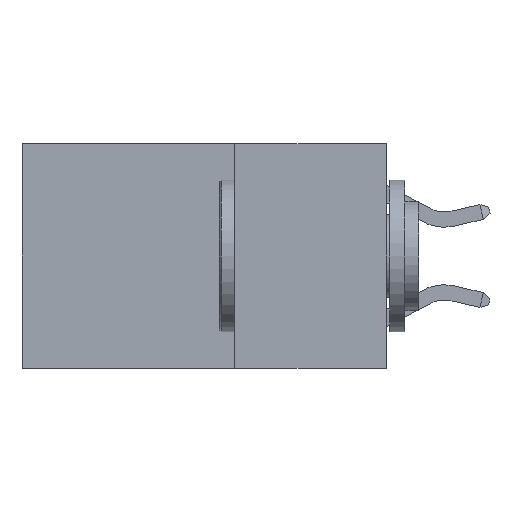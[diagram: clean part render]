
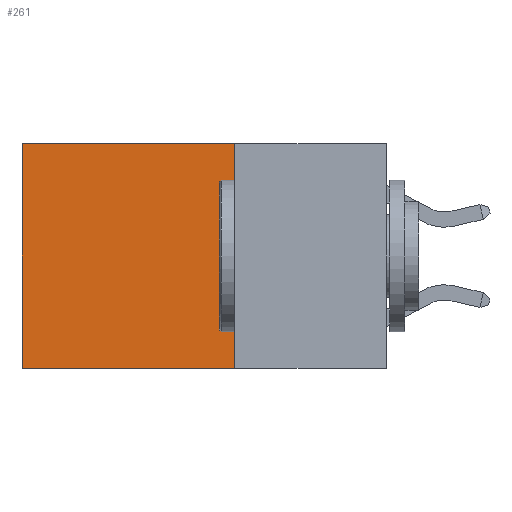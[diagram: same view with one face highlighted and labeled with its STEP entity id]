
A CAD part, left-side view. The second image highlights one B-rep face of the part: STEP entity #261.
In plain terms, the highlighted planar face has unit normal (-1, 0, 0).
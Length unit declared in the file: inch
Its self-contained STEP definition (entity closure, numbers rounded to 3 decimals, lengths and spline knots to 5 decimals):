
#239 = CARTESIAN_POINT ( 'NONE',  ( 0.2625, 0.25, 0. ) ) ;
#261 = ADVANCED_FACE ( 'NONE', ( #4625 ), #5172, .F. ) ;
#1072 = VERTEX_POINT ( 'NONE', #8685 ) ;
#1310 = CARTESIAN_POINT ( 'NONE',  ( 0.2625, 0.6, 0. ) ) ;
#2101 = ORIENTED_EDGE ( 'NONE', *, *, #4973, .T. ) ;
#2109 = LINE ( 'NONE', #1310, #5871 ) ;
#2113 = ORIENTED_EDGE ( 'NONE', *, *, #4403, .F. ) ;
#2127 = ORIENTED_EDGE ( 'NONE', *, *, #2894, .F. ) ;
#2142 = ORIENTED_EDGE ( 'NONE', *, *, #4679, .T. ) ;
#2281 = DIRECTION ( 'NONE',  ( 0., 0., -1. ) ) ;
#2725 = CARTESIAN_POINT ( 'NONE',  ( 0.2625, 0.6, 0. ) ) ;
#2894 = EDGE_CURVE ( 'NONE', #7991, #3366, #8858, .T. ) ;
#3233 = DIRECTION ( 'NONE',  ( 0., 1., 0. ) ) ;
#3366 = VERTEX_POINT ( 'NONE', #7123 ) ;
#3646 = LINE ( 'NONE', #7152, #8243 ) ;
#4132 = LINE ( 'NONE', #7445, #8565 ) ;
#4403 = EDGE_CURVE ( 'NONE', #3366, #1072, #3646, .T. ) ;
#4625 = FACE_OUTER_BOUND ( 'NONE', #6244, .T. ) ;
#4679 = EDGE_CURVE ( 'NONE', #7991, #5270, #4132, .T. ) ;
#4850 = CARTESIAN_POINT ( 'NONE',  ( 0.2625, 0.25, 0. ) ) ;
#4965 = DIRECTION ( 'NONE',  ( 0., 0., -1. ) ) ;
#4973 = EDGE_CURVE ( 'NONE', #5270, #1072, #2109, .T. ) ;
#5033 = DIRECTION ( 'NONE',  ( 0., 1., 0. ) ) ;
#5123 = AXIS2_PLACEMENT_3D ( 'NONE', #5503, #5298, #7067 ) ;
#5172 = PLANE ( 'NONE',  #5123 ) ;
#5270 = VERTEX_POINT ( 'NONE', #2725 ) ;
#5298 = DIRECTION ( 'NONE',  ( 1., 0., 0. ) ) ;
#5503 = CARTESIAN_POINT ( 'NONE',  ( 0.2625, 0.25, 0. ) ) ;
#5871 = VECTOR ( 'NONE', #2281, 39.37008 ) ;
#6244 = EDGE_LOOP ( 'NONE', ( #2101, #2113, #2127, #2142 ) ) ;
#7067 = DIRECTION ( 'NONE',  ( 0., 0., -1. ) ) ;
#7123 = CARTESIAN_POINT ( 'NONE',  ( 0.2625, 0.25, -0.37 ) ) ;
#7152 = CARTESIAN_POINT ( 'NONE',  ( 0.2625, 0.25, -0.37 ) ) ;
#7406 = VECTOR ( 'NONE', #4965, 39.37008 ) ;
#7445 = CARTESIAN_POINT ( 'NONE',  ( 0.2625, 0.25, 0. ) ) ;
#7991 = VERTEX_POINT ( 'NONE', #239 ) ;
#8243 = VECTOR ( 'NONE', #3233, 39.37008 ) ;
#8565 = VECTOR ( 'NONE', #5033, 39.37008 ) ;
#8685 = CARTESIAN_POINT ( 'NONE',  ( 0.2625, 0.6, -0.37 ) ) ;
#8858 = LINE ( 'NONE', #4850, #7406 ) ;
